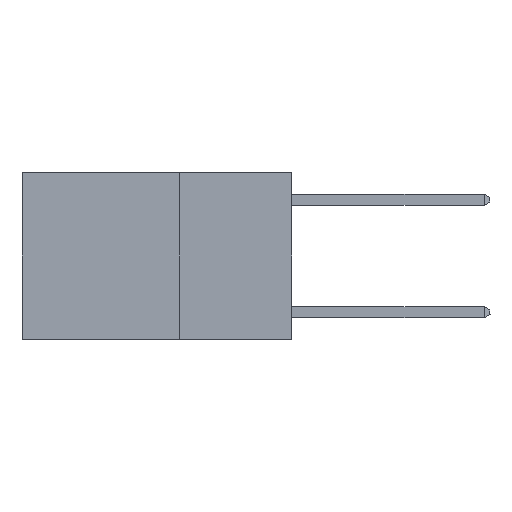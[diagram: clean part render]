
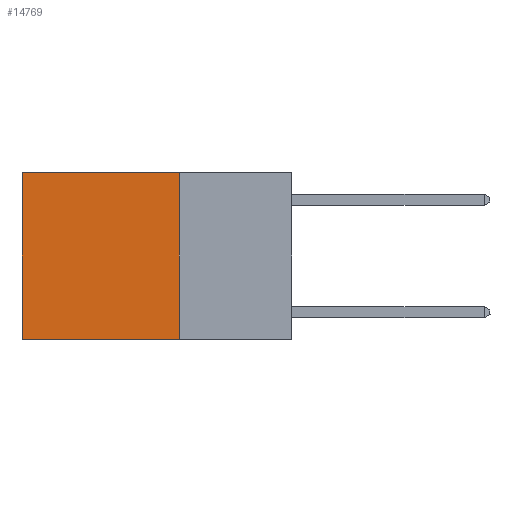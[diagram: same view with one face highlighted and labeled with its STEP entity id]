
A CAD part, left-side view. The second image highlights one B-rep face of the part: STEP entity #14769.
In plain terms, the highlighted planar face has unit normal (-1, 0, 0).
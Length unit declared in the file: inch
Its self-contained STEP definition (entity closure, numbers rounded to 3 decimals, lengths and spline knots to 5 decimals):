
#187 = FACE_OUTER_BOUND ( 'NONE', #7979, .T. ) ;
#246 = VECTOR ( 'NONE', #1934, 39.37008 ) ;
#311 = VERTEX_POINT ( 'NONE', #703 ) ;
#526 = DIRECTION ( 'NONE',  ( 0., 0., -1. ) ) ;
#703 = CARTESIAN_POINT ( 'NONE',  ( 0.2625, 0.6, -0.37 ) ) ;
#1193 = CARTESIAN_POINT ( 'NONE',  ( 0.2625, 0.25, -0.37 ) ) ;
#1934 = DIRECTION ( 'NONE',  ( 0., 1., 0. ) ) ;
#2280 = ORIENTED_EDGE ( 'NONE', *, *, #13329, .T. ) ;
#2525 = VERTEX_POINT ( 'NONE', #5526 ) ;
#3829 = DIRECTION ( 'NONE',  ( 0., 0., -1. ) ) ;
#4739 = LINE ( 'NONE', #12483, #9062 ) ;
#5317 = LINE ( 'NONE', #15245, #13991 ) ;
#5526 = CARTESIAN_POINT ( 'NONE',  ( 0.2625, 0.25, 0. ) ) ;
#6056 = VERTEX_POINT ( 'NONE', #1193 ) ;
#7596 = DIRECTION ( 'NONE',  ( 0., 0., -1. ) ) ;
#7733 = DIRECTION ( 'NONE',  ( 0., 1., 0. ) ) ;
#7979 = EDGE_LOOP ( 'NONE', ( #2280, #17535, #10712, #12896 ) ) ;
#8146 = EDGE_CURVE ( 'NONE', #6056, #311, #17126, .T. ) ;
#8722 = CARTESIAN_POINT ( 'NONE',  ( 0.2625, 0.25, 0. ) ) ;
#9062 = VECTOR ( 'NONE', #7596, 39.37008 ) ;
#9370 = CARTESIAN_POINT ( 'NONE',  ( 0.2625, 0.25, 0. ) ) ;
#10389 = DIRECTION ( 'NONE',  ( 1., 0., 0. ) ) ;
#10712 = ORIENTED_EDGE ( 'NONE', *, *, #17579, .F. ) ;
#10906 = CARTESIAN_POINT ( 'NONE',  ( 0.2625, 0.6, 0. ) ) ;
#12483 = CARTESIAN_POINT ( 'NONE',  ( 0.2625, 0.6, 0. ) ) ;
#12896 = ORIENTED_EDGE ( 'NONE', *, *, #16997, .T. ) ;
#13329 = EDGE_CURVE ( 'NONE', #13945, #311, #4739, .T. ) ;
#13945 = VERTEX_POINT ( 'NONE', #10906 ) ;
#13991 = VECTOR ( 'NONE', #3829, 39.37008 ) ;
#14769 = ADVANCED_FACE ( 'NONE', ( #187 ), #18325, .F. ) ;
#15245 = CARTESIAN_POINT ( 'NONE',  ( 0.2625, 0.25, 0. ) ) ;
#16244 = VECTOR ( 'NONE', #7733, 39.37008 ) ;
#16624 = CARTESIAN_POINT ( 'NONE',  ( 0.2625, 0.25, -0.37 ) ) ;
#16997 = EDGE_CURVE ( 'NONE', #2525, #13945, #19704, .T. ) ;
#17126 = LINE ( 'NONE', #16624, #246 ) ;
#17535 = ORIENTED_EDGE ( 'NONE', *, *, #8146, .F. ) ;
#17579 = EDGE_CURVE ( 'NONE', #2525, #6056, #5317, .T. ) ;
#18325 = PLANE ( 'NONE',  #19192 ) ;
#19192 = AXIS2_PLACEMENT_3D ( 'NONE', #8722, #10389, #526 ) ;
#19704 = LINE ( 'NONE', #9370, #16244 ) ;
